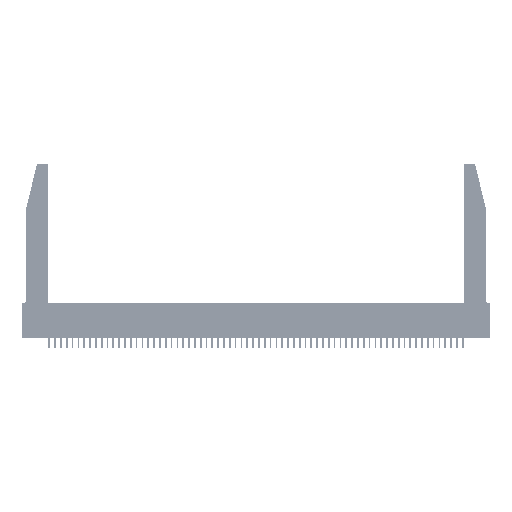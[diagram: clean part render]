
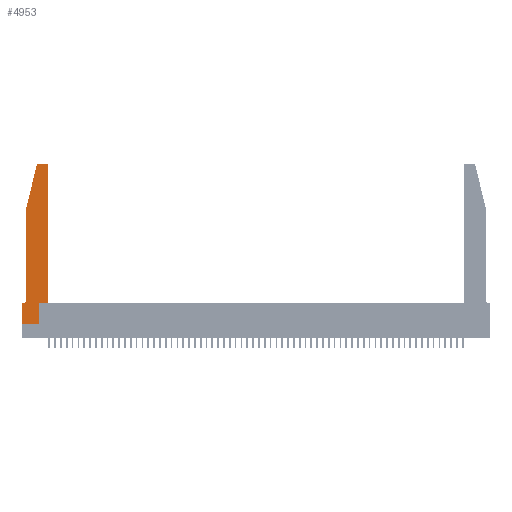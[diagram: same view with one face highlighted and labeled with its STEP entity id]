
A CAD part, top view. The second image highlights one B-rep face of the part: STEP entity #4953.
In plain terms, the highlighted planar face has unit normal (0, 0, 1).
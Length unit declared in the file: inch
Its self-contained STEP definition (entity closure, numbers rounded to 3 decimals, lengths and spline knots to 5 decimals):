
#5 = EDGE_CURVE ( 'NONE', #21245, #57234, #41543, .T. ) ;
#410 = CARTESIAN_POINT ( 'NONE',  ( 0., 0., 0.37 ) ) ;
#942 = CARTESIAN_POINT ( 'NONE',  ( 0.284, 2.75, 0.37 ) ) ;
#1396 = VERTEX_POINT ( 'NONE', #410 ) ;
#1974 = VERTEX_POINT ( 'NONE', #21732 ) ;
#2050 = CARTESIAN_POINT ( 'NONE',  ( 0.4505, 0.35, 0.37 ) ) ;
#2877 = VECTOR ( 'NONE', #12284, 39.37008 ) ;
#2993 = EDGE_CURVE ( 'NONE', #36619, #47913, #23801, .T. ) ;
#3418 = CARTESIAN_POINT ( 'NONE',  ( 0.0755, 0.35, 0.37 ) ) ;
#3844 = AXIS2_PLACEMENT_3D ( 'NONE', #5117, #31645, #53980 ) ;
#3863 = CIRCLE ( 'NONE', #36722, 0.07 ) ;
#4953 = ADVANCED_FACE ( 'NONE', ( #9874 ), #11893, .T. ) ;
#5117 = CARTESIAN_POINT ( 'NONE',  ( 0.4205, 2.72, 0.37 ) ) ;
#5915 = DIRECTION ( 'NONE',  ( 0., 0., -1. ) ) ;
#6717 = LINE ( 'NONE', #3418, #18455 ) ;
#6730 = EDGE_CURVE ( 'NONE', #57234, #36619, #46519, .T. ) ;
#7280 = CARTESIAN_POINT ( 'NONE',  ( 0.284, 2.72, 0.37 ) ) ;
#7848 = ORIENTED_EDGE ( 'NONE', *, *, #5, .T. ) ;
#8247 = ORIENTED_EDGE ( 'NONE', *, *, #15650, .T. ) ;
#9874 = FACE_OUTER_BOUND ( 'NONE', #34814, .T. ) ;
#10071 = DIRECTION ( 'NONE',  ( 0., -1., 0. ) ) ;
#10893 = CARTESIAN_POINT ( 'NONE',  ( 0., 0., 0.37 ) ) ;
#11693 = DIRECTION ( 'NONE',  ( 1., 0., 0. ) ) ;
#11893 = PLANE ( 'NONE',  #12085 ) ;
#12085 = AXIS2_PLACEMENT_3D ( 'NONE', #43004, #47452, #20796 ) ;
#12284 = DIRECTION ( 'NONE',  ( 0., 1., 0. ) ) ;
#13406 = VECTOR ( 'NONE', #50752, 39.37008 ) ;
#14331 = EDGE_CURVE ( 'NONE', #22921, #34478, #16299, .T. ) ;
#15650 = EDGE_CURVE ( 'NONE', #54508, #1396, #55169, .T. ) ;
#15735 = CARTESIAN_POINT ( 'NONE',  ( 0.4505, 0.35, 0.37 ) ) ;
#16299 = LINE ( 'NONE', #28114, #38580 ) ;
#18455 = VECTOR ( 'NONE', #29887, 39.37008 ) ;
#19650 = CARTESIAN_POINT ( 'NONE',  ( 0.2865, 0.35, 0.37 ) ) ;
#19708 = VECTOR ( 'NONE', #46459, 39.37008 ) ;
#20667 = CARTESIAN_POINT ( 'NONE',  ( 0.0755, 2., 0.37 ) ) ;
#20796 = DIRECTION ( 'NONE',  ( 1., 0., 0. ) ) ;
#21245 = VERTEX_POINT ( 'NONE', #30167 ) ;
#21732 = CARTESIAN_POINT ( 'NONE',  ( 0.0055, 0.35, 0.37 ) ) ;
#21854 = DIRECTION ( 'NONE',  ( 1., 0., 0. ) ) ;
#21864 = VERTEX_POINT ( 'NONE', #35575 ) ;
#22663 = EDGE_CURVE ( 'NONE', #47913, #22921, #24555, .T. ) ;
#22829 = VECTOR ( 'NONE', #56659, 39.37008 ) ;
#22921 = VERTEX_POINT ( 'NONE', #20667 ) ;
#23428 = ORIENTED_EDGE ( 'NONE', *, *, #25879, .T. ) ;
#23673 = ORIENTED_EDGE ( 'NONE', *, *, #51832, .T. ) ;
#23787 = LINE ( 'NONE', #19650, #13406 ) ;
#23801 = CIRCLE ( 'NONE', #24635, 0.03 ) ;
#24024 = DIRECTION ( 'NONE',  ( 1., 0., 0. ) ) ;
#24555 = LINE ( 'NONE', #28082, #46855 ) ;
#24635 = AXIS2_PLACEMENT_3D ( 'NONE', #7280, #38318, #11693 ) ;
#25645 = CARTESIAN_POINT ( 'NONE',  ( 0.0755, 0.42, 0.37 ) ) ;
#25879 = EDGE_CURVE ( 'NONE', #36279, #21245, #50020, .T. ) ;
#26281 = LINE ( 'NONE', #35296, #48556 ) ;
#27239 = ORIENTED_EDGE ( 'NONE', *, *, #14331, .T. ) ;
#28082 = CARTESIAN_POINT ( 'NONE',  ( 0.0755, 2., 0.37 ) ) ;
#28114 = CARTESIAN_POINT ( 'NONE',  ( 0.0755, 2., 0.37 ) ) ;
#29082 = EDGE_CURVE ( 'NONE', #34478, #1974, #3863, .T. ) ;
#29887 = DIRECTION ( 'NONE',  ( -1., 0., 0. ) ) ;
#30025 = CARTESIAN_POINT ( 'NONE',  ( 0.2605, 2.75, 0.37 ) ) ;
#30167 = CARTESIAN_POINT ( 'NONE',  ( 0.4505, 2.72, 0.37 ) ) ;
#31645 = DIRECTION ( 'NONE',  ( 0., 0., 1. ) ) ;
#32364 = ORIENTED_EDGE ( 'NONE', *, *, #46233, .T. ) ;
#32467 = CARTESIAN_POINT ( 'NONE',  ( 0.0055, 0.42, 0.37 ) ) ;
#32551 = DIRECTION ( 'NONE',  ( -0.239, -0.971, 0. ) ) ;
#34189 = EDGE_CURVE ( 'NONE', #21864, #36028, #23787, .T. ) ;
#34336 = CARTESIAN_POINT ( 'NONE',  ( 0.25487, 2.72718, 0.37 ) ) ;
#34478 = VERTEX_POINT ( 'NONE', #25645 ) ;
#34814 = EDGE_LOOP ( 'NONE', ( #44729, #56989, #45690, #27239, #35548, #32364, #8247, #23673, #54126, #46411, #23428, #7848 ) ) ;
#34852 = CARTESIAN_POINT ( 'NONE',  ( 0., 0.35, 0.37 ) ) ;
#35296 = CARTESIAN_POINT ( 'NONE',  ( 0., 0., 0.37 ) ) ;
#35548 = ORIENTED_EDGE ( 'NONE', *, *, #29082, .T. ) ;
#35575 = CARTESIAN_POINT ( 'NONE',  ( 0.2865, 0., 0.37 ) ) ;
#36028 = VERTEX_POINT ( 'NONE', #40672 ) ;
#36279 = VERTEX_POINT ( 'NONE', #15735 ) ;
#36619 = VERTEX_POINT ( 'NONE', #942 ) ;
#36722 = AXIS2_PLACEMENT_3D ( 'NONE', #32467, #5915, #36934 ) ;
#36934 = DIRECTION ( 'NONE',  ( -1., 0., 0. ) ) ;
#37011 = CARTESIAN_POINT ( 'NONE',  ( 0.4205, 2.75, 0.37 ) ) ;
#38318 = DIRECTION ( 'NONE',  ( 0., 0., 1. ) ) ;
#38580 = VECTOR ( 'NONE', #10071, 39.37008 ) ;
#40672 = CARTESIAN_POINT ( 'NONE',  ( 0.2865, 0.35, 0.37 ) ) ;
#41543 = CIRCLE ( 'NONE', #3844, 0.03 ) ;
#43004 = CARTESIAN_POINT ( 'NONE',  ( 0., 0.35, 0.37 ) ) ;
#44729 = ORIENTED_EDGE ( 'NONE', *, *, #6730, .T. ) ;
#45690 = ORIENTED_EDGE ( 'NONE', *, *, #22663, .T. ) ;
#46233 = EDGE_CURVE ( 'NONE', #1974, #54508, #6717, .T. ) ;
#46411 = ORIENTED_EDGE ( 'NONE', *, *, #53497, .T. ) ;
#46459 = DIRECTION ( 'NONE',  ( 0., -1., 0. ) ) ;
#46519 = LINE ( 'NONE', #30025, #22829 ) ;
#46855 = VECTOR ( 'NONE', #32551, 39.37008 ) ;
#47452 = DIRECTION ( 'NONE',  ( 0., 0., 1. ) ) ;
#47836 = CARTESIAN_POINT ( 'NONE',  ( 0.4505, 0.35, 0.37 ) ) ;
#47913 = VERTEX_POINT ( 'NONE', #34336 ) ;
#48556 = VECTOR ( 'NONE', #21854, 39.37008 ) ;
#50020 = LINE ( 'NONE', #47836, #2877 ) ;
#50752 = DIRECTION ( 'NONE',  ( 0., 1., 0. ) ) ;
#51832 = EDGE_CURVE ( 'NONE', #1396, #21864, #26281, .T. ) ;
#53497 = EDGE_CURVE ( 'NONE', #36028, #36279, #55283, .T. ) ;
#53895 = VECTOR ( 'NONE', #24024, 39.37008 ) ;
#53980 = DIRECTION ( 'NONE',  ( 1., 0., 0. ) ) ;
#54126 = ORIENTED_EDGE ( 'NONE', *, *, #34189, .T. ) ;
#54508 = VERTEX_POINT ( 'NONE', #34852 ) ;
#55169 = LINE ( 'NONE', #10893, #19708 ) ;
#55283 = LINE ( 'NONE', #2050, #53895 ) ;
#56659 = DIRECTION ( 'NONE',  ( -1., 0., 0. ) ) ;
#56989 = ORIENTED_EDGE ( 'NONE', *, *, #2993, .T. ) ;
#57234 = VERTEX_POINT ( 'NONE', #37011 ) ;
